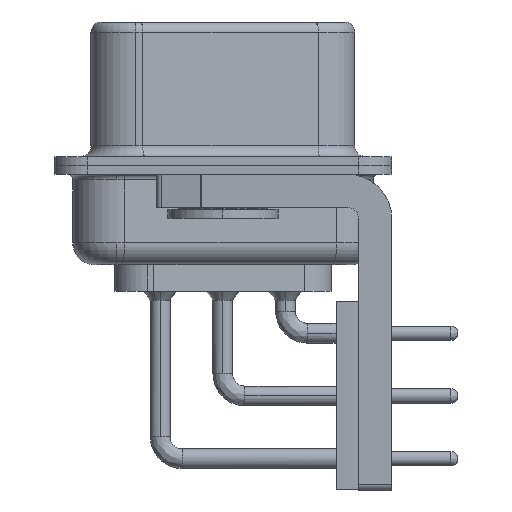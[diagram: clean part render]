
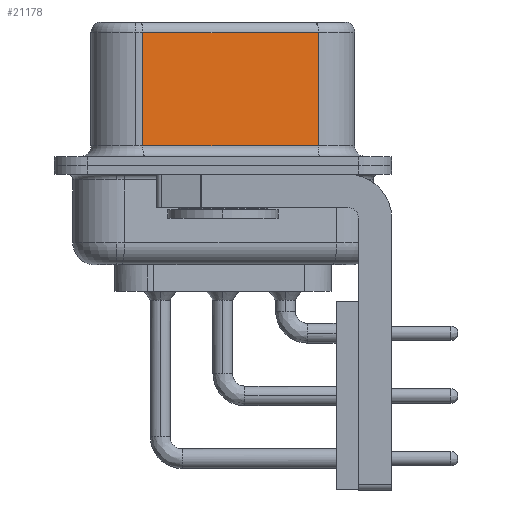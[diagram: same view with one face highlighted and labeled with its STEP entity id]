
A CAD part, left-side view. The second image highlights one B-rep face of the part: STEP entity #21178.
In plain terms, the highlighted planar face has unit normal (-0.985, -0.174, 0).
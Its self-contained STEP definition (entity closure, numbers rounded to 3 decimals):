
#702 = FACE_OUTER_BOUND ( 'NONE', #949, .T. ) ;
#949 = EDGE_LOOP ( 'NONE', ( #31602, #7864, #17533, #25551 ) ) ;
#1424 = VERTEX_POINT ( 'NONE', #9048 ) ;
#1706 = AXIS2_PLACEMENT_3D ( 'NONE', #5414, #34574, #15308 ) ;
#2106 = PLANE ( 'NONE',  #1706 ) ;
#3238 = DIRECTION ( 'NONE',  ( 0., 0., -1. ) ) ;
#3770 = VECTOR ( 'NONE', #3238, 1000. ) ;
#5414 = CARTESIAN_POINT ( 'NONE',  ( 5.132, -4.322, 6.52 ) ) ;
#6302 = LINE ( 'NONE', #7638, #30101 ) ;
#7159 = CARTESIAN_POINT ( 'NONE',  ( 5.132, -4.322, 0.9 ) ) ;
#7638 = CARTESIAN_POINT ( 'NONE',  ( 5.132, -4.322, 6.02 ) ) ;
#7864 = ORIENTED_EDGE ( 'NONE', *, *, #38641, .T. ) ;
#8164 = CARTESIAN_POINT ( 'NONE',  ( 5.132, -4.322, 0.9 ) ) ;
#8788 = EDGE_CURVE ( 'NONE', #1424, #17282, #37660, .T. ) ;
#9048 = CARTESIAN_POINT ( 'NONE',  ( 3.73, 3.628, 0.9 ) ) ;
#9418 = DIRECTION ( 'NONE',  ( 0., 0., -1. ) ) ;
#10893 = DIRECTION ( 'NONE',  ( -0.174, 0.985, 0. ) ) ;
#11461 = CARTESIAN_POINT ( 'NONE',  ( 5.132, -4.322, 6.02 ) ) ;
#12869 = CARTESIAN_POINT ( 'NONE',  ( 5.132, -4.322, 6.52 ) ) ;
#12946 = VECTOR ( 'NONE', #33997, 1000. ) ;
#15308 = DIRECTION ( 'NONE',  ( -0.174, 0.985, 0. ) ) ;
#17282 = VERTEX_POINT ( 'NONE', #7159 ) ;
#17533 = ORIENTED_EDGE ( 'NONE', *, *, #40181, .T. ) ;
#19569 = EDGE_CURVE ( 'NONE', #37368, #17282, #19686, .T. ) ;
#19686 = LINE ( 'NONE', #12869, #27214 ) ;
#20107 = LINE ( 'NONE', #22792, #3770 ) ;
#21178 = ADVANCED_FACE ( 'NONE', ( #702 ), #2106, .F. ) ;
#22792 = CARTESIAN_POINT ( 'NONE',  ( 3.73, 3.628, 6.52 ) ) ;
#25551 = ORIENTED_EDGE ( 'NONE', *, *, #8788, .T. ) ;
#27214 = VECTOR ( 'NONE', #9418, 1000. ) ;
#30101 = VECTOR ( 'NONE', #10893, 1000. ) ;
#31602 = ORIENTED_EDGE ( 'NONE', *, *, #19569, .F. ) ;
#33997 = DIRECTION ( 'NONE',  ( 0.174, -0.985, 0. ) ) ;
#34574 = DIRECTION ( 'NONE',  ( 0.985, 0.174, 0. ) ) ;
#35372 = VERTEX_POINT ( 'NONE', #35921 ) ;
#35921 = CARTESIAN_POINT ( 'NONE',  ( 3.73, 3.628, 6.02 ) ) ;
#37368 = VERTEX_POINT ( 'NONE', #11461 ) ;
#37660 = LINE ( 'NONE', #8164, #12946 ) ;
#38641 = EDGE_CURVE ( 'NONE', #37368, #35372, #6302, .T. ) ;
#40181 = EDGE_CURVE ( 'NONE', #35372, #1424, #20107, .T. ) ;
